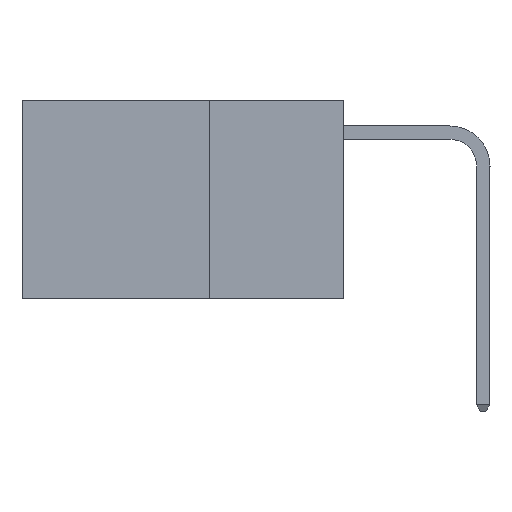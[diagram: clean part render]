
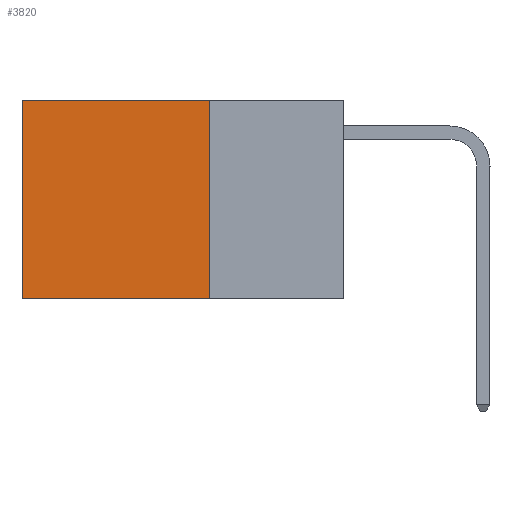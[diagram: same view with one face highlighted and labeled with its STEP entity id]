
A CAD part, left-side view. The second image highlights one B-rep face of the part: STEP entity #3820.
In plain terms, the highlighted planar face has unit normal (-1, 0, 0).
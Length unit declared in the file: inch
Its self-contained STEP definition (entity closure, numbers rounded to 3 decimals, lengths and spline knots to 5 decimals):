
#1268 = DIRECTION ( 'NONE',  ( 1., 0., 0. ) ) ;
#1281 = DIRECTION ( 'NONE',  ( 0., 0., -1. ) ) ;
#1370 = CARTESIAN_POINT ( 'NONE',  ( 0.2625, 0.25, 0. ) ) ;
#1578 = DIRECTION ( 'NONE',  ( 0., 1., 0. ) ) ;
#1647 = CARTESIAN_POINT ( 'NONE',  ( 0.2625, 0.25, 0. ) ) ;
#1666 = VERTEX_POINT ( 'NONE', #6487 ) ;
#2252 = VECTOR ( 'NONE', #9162, 39.37008 ) ;
#2471 = EDGE_CURVE ( 'NONE', #7500, #11721, #6364, .T. ) ;
#2664 = CARTESIAN_POINT ( 'NONE',  ( 0.2625, 0.25, 0. ) ) ;
#2676 = ORIENTED_EDGE ( 'NONE', *, *, #3123, .F. ) ;
#2861 = CARTESIAN_POINT ( 'NONE',  ( 0.2625, 0.25, -0.37 ) ) ;
#3009 = ORIENTED_EDGE ( 'NONE', *, *, #2471, .T. ) ;
#3123 = EDGE_CURVE ( 'NONE', #8329, #1666, #13591, .T. ) ;
#3820 = ADVANCED_FACE ( 'NONE', ( #10250 ), #4777, .F. ) ;
#4126 = DIRECTION ( 'NONE',  ( 0., 0., -1. ) ) ;
#4777 = PLANE ( 'NONE',  #13103 ) ;
#5175 = LINE ( 'NONE', #11722, #10622 ) ;
#5334 = VECTOR ( 'NONE', #10698, 39.37008 ) ;
#5546 = ORIENTED_EDGE ( 'NONE', *, *, #10083, .F. ) ;
#6364 = LINE ( 'NONE', #1370, #9264 ) ;
#6487 = CARTESIAN_POINT ( 'NONE',  ( 0.2625, 0.6, -0.37 ) ) ;
#6724 = EDGE_LOOP ( 'NONE', ( #7788, #2676, #5546, #3009 ) ) ;
#7500 = VERTEX_POINT ( 'NONE', #11271 ) ;
#7788 = ORIENTED_EDGE ( 'NONE', *, *, #13050, .T. ) ;
#8329 = VERTEX_POINT ( 'NONE', #2861 ) ;
#9162 = DIRECTION ( 'NONE',  ( 0., 0., -1. ) ) ;
#9264 = VECTOR ( 'NONE', #1578, 39.37008 ) ;
#10083 = EDGE_CURVE ( 'NONE', #7500, #8329, #11240, .T. ) ;
#10250 = FACE_OUTER_BOUND ( 'NONE', #6724, .T. ) ;
#10563 = CARTESIAN_POINT ( 'NONE',  ( 0.2625, 0.25, -0.37 ) ) ;
#10622 = VECTOR ( 'NONE', #4126, 39.37008 ) ;
#10698 = DIRECTION ( 'NONE',  ( 0., 1., 0. ) ) ;
#11240 = LINE ( 'NONE', #2664, #2252 ) ;
#11271 = CARTESIAN_POINT ( 'NONE',  ( 0.2625, 0.25, 0. ) ) ;
#11721 = VERTEX_POINT ( 'NONE', #13887 ) ;
#11722 = CARTESIAN_POINT ( 'NONE',  ( 0.2625, 0.6, 0. ) ) ;
#13050 = EDGE_CURVE ( 'NONE', #11721, #1666, #5175, .T. ) ;
#13103 = AXIS2_PLACEMENT_3D ( 'NONE', #1647, #1268, #1281 ) ;
#13591 = LINE ( 'NONE', #10563, #5334 ) ;
#13887 = CARTESIAN_POINT ( 'NONE',  ( 0.2625, 0.6, 0. ) ) ;
